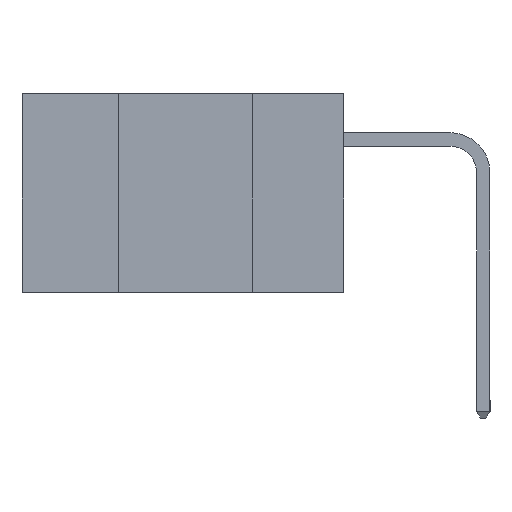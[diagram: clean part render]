
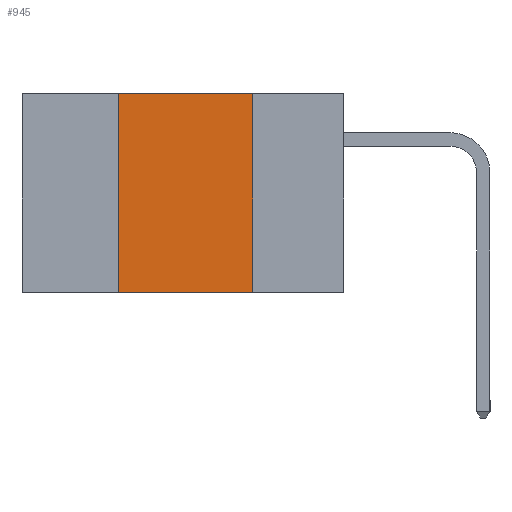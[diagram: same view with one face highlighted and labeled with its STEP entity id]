
A CAD part, left-side view. The second image highlights one B-rep face of the part: STEP entity #945.
In plain terms, the highlighted planar face has unit normal (-1, 0, 0).
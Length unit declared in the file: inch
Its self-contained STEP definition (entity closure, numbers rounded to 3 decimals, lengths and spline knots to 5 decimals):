
#639 = CARTESIAN_POINT ( 'NONE',  ( 0., 0.6, 0. ) ) ;
#767 = AXIS2_PLACEMENT_3D ( 'NONE', #639, #13843, #12637 ) ;
#945 = ADVANCED_FACE ( 'NONE', ( #8856 ), #11566, .F. ) ;
#1823 = DIRECTION ( 'NONE',  ( 0., 0., -1. ) ) ;
#2187 = LINE ( 'NONE', #13802, #13648 ) ;
#2570 = VECTOR ( 'NONE', #1823, 39.37008 ) ;
#3267 = LINE ( 'NONE', #11976, #7941 ) ;
#3438 = LINE ( 'NONE', #9923, #2570 ) ;
#3615 = EDGE_CURVE ( 'NONE', #5138, #7517, #3438, .T. ) ;
#4666 = EDGE_LOOP ( 'NONE', ( #13466, #8927, #10642, #11035 ) ) ;
#4668 = VERTEX_POINT ( 'NONE', #7771 ) ;
#4692 = CARTESIAN_POINT ( 'NONE',  ( 0., 0.42, -0.37 ) ) ;
#4957 = EDGE_CURVE ( 'NONE', #9381, #4668, #2187, .T. ) ;
#5138 = VERTEX_POINT ( 'NONE', #7654 ) ;
#5334 = DIRECTION ( 'NONE',  ( 0., -1., 0. ) ) ;
#6363 = VECTOR ( 'NONE', #9142, 39.37008 ) ;
#7402 = LINE ( 'NONE', #11347, #6363 ) ;
#7517 = VERTEX_POINT ( 'NONE', #9834 ) ;
#7654 = CARTESIAN_POINT ( 'NONE',  ( 0., 0.17, 0. ) ) ;
#7771 = CARTESIAN_POINT ( 'NONE',  ( 0., 0.42, 0. ) ) ;
#7941 = VECTOR ( 'NONE', #5334, 39.37008 ) ;
#8250 = DIRECTION ( 'NONE',  ( 0., 0., 1. ) ) ;
#8856 = FACE_OUTER_BOUND ( 'NONE', #4666, .T. ) ;
#8927 = ORIENTED_EDGE ( 'NONE', *, *, #13016, .F. ) ;
#9142 = DIRECTION ( 'NONE',  ( 0., -1., 0. ) ) ;
#9381 = VERTEX_POINT ( 'NONE', #4692 ) ;
#9834 = CARTESIAN_POINT ( 'NONE',  ( 0., 0.17, -0.37 ) ) ;
#9923 = CARTESIAN_POINT ( 'NONE',  ( 0., 0.17, -0.37 ) ) ;
#10110 = EDGE_CURVE ( 'NONE', #9381, #7517, #7402, .T. ) ;
#10642 = ORIENTED_EDGE ( 'NONE', *, *, #4957, .F. ) ;
#11035 = ORIENTED_EDGE ( 'NONE', *, *, #10110, .T. ) ;
#11347 = CARTESIAN_POINT ( 'NONE',  ( 0., 0.6, -0.37 ) ) ;
#11566 = PLANE ( 'NONE',  #767 ) ;
#11976 = CARTESIAN_POINT ( 'NONE',  ( 0., 0.6, 0. ) ) ;
#12637 = DIRECTION ( 'NONE',  ( 0., 0., -1. ) ) ;
#13016 = EDGE_CURVE ( 'NONE', #4668, #5138, #3267, .T. ) ;
#13466 = ORIENTED_EDGE ( 'NONE', *, *, #3615, .F. ) ;
#13648 = VECTOR ( 'NONE', #8250, 39.37008 ) ;
#13802 = CARTESIAN_POINT ( 'NONE',  ( 0., 0.42, -0.37 ) ) ;
#13843 = DIRECTION ( 'NONE',  ( 1., 0., 0. ) ) ;
